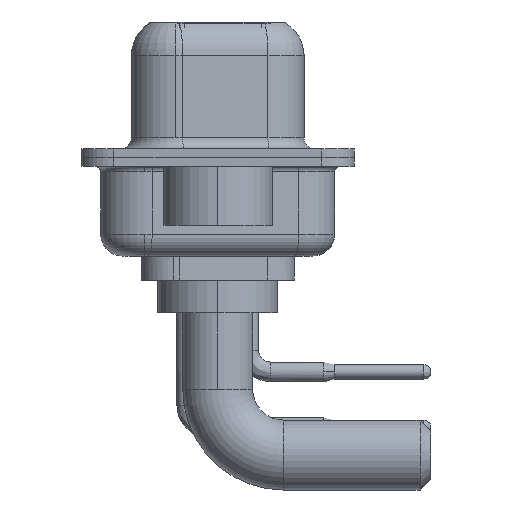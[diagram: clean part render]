
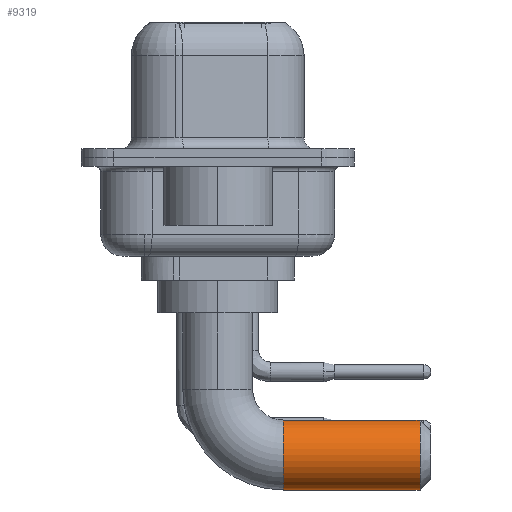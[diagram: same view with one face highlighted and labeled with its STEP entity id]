
A CAD part, left-side view. The second image highlights one B-rep face of the part: STEP entity #9319.
In plain terms, the highlighted cylindrical face has radius 1.6 mm (diameter 3.2 mm), a partial arc.
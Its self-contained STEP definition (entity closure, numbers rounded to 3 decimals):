
#803 = CARTESIAN_POINT ( 'NONE',  ( 0., -3., -6.5 ) ) ;
#983 = DIRECTION ( 'NONE',  ( 0., 1., 0. ) ) ;
#1388 = EDGE_CURVE ( 'NONE', #18819, #10625, #2335, .T. ) ;
#2335 = LINE ( 'NONE', #11753, #11101 ) ;
#2569 = CARTESIAN_POINT ( 'NONE',  ( 0., -3., -8.1 ) ) ;
#2604 = EDGE_CURVE ( 'NONE', #12490, #14874, #17315, .T. ) ;
#2717 = CYLINDRICAL_SURFACE ( 'NONE', #2975, 1.6 ) ;
#2975 = AXIS2_PLACEMENT_3D ( 'NONE', #803, #11573, #9937 ) ;
#3113 = EDGE_LOOP ( 'NONE', ( #14633, #6353, #15733, #12248 ) ) ;
#3656 = FACE_OUTER_BOUND ( 'NONE', #3113, .T. ) ;
#4587 = EDGE_CURVE ( 'NONE', #10625, #14874, #14179, .T. ) ;
#4609 = VECTOR ( 'NONE', #6650, 1000. ) ;
#5911 = AXIS2_PLACEMENT_3D ( 'NONE', #18859, #15794, #10660 ) ;
#6353 = ORIENTED_EDGE ( 'NONE', *, *, #18960, .T. ) ;
#6650 = DIRECTION ( 'NONE',  ( 0., -1., 0. ) ) ;
#6944 = DIRECTION ( 'NONE',  ( 0., -1., 0. ) ) ;
#7885 = CARTESIAN_POINT ( 'NONE',  ( 0., -3., -4.9 ) ) ;
#9319 = ADVANCED_FACE ( 'NONE', ( #3656 ), #2717, .T. ) ;
#9937 = DIRECTION ( 'NONE',  ( 0., 0., -1. ) ) ;
#10315 = DIRECTION ( 'NONE',  ( 0., 0., -1. ) ) ;
#10625 = VERTEX_POINT ( 'NONE', #16596 ) ;
#10660 = DIRECTION ( 'NONE',  ( -1., 0., 0. ) ) ;
#11101 = VECTOR ( 'NONE', #6944, 1000. ) ;
#11573 = DIRECTION ( 'NONE',  ( 0., -1., 0. ) ) ;
#11753 = CARTESIAN_POINT ( 'NONE',  ( 0., -3., -8.1 ) ) ;
#11893 = AXIS2_PLACEMENT_3D ( 'NONE', #13393, #983, #10315 ) ;
#12248 = ORIENTED_EDGE ( 'NONE', *, *, #4587, .T. ) ;
#12490 = VERTEX_POINT ( 'NONE', #19795 ) ;
#13393 = CARTESIAN_POINT ( 'NONE',  ( 0., -9.25, -6.5 ) ) ;
#14179 = CIRCLE ( 'NONE', #11893, 1.6 ) ;
#14633 = ORIENTED_EDGE ( 'NONE', *, *, #2604, .F. ) ;
#14874 = VERTEX_POINT ( 'NONE', #15286 ) ;
#15286 = CARTESIAN_POINT ( 'NONE',  ( 0., -9.25, -4.9 ) ) ;
#15733 = ORIENTED_EDGE ( 'NONE', *, *, #1388, .T. ) ;
#15794 = DIRECTION ( 'NONE',  ( 0., -1., 0. ) ) ;
#16596 = CARTESIAN_POINT ( 'NONE',  ( 0., -9.25, -8.1 ) ) ;
#16725 = CIRCLE ( 'NONE', #5911, 1.6 ) ;
#17315 = LINE ( 'NONE', #7885, #4609 ) ;
#18819 = VERTEX_POINT ( 'NONE', #2569 ) ;
#18859 = CARTESIAN_POINT ( 'NONE',  ( 0., -3., -6.5 ) ) ;
#18960 = EDGE_CURVE ( 'NONE', #12490, #18819, #16725, .T. ) ;
#19795 = CARTESIAN_POINT ( 'NONE',  ( 0., -3., -4.9 ) ) ;
